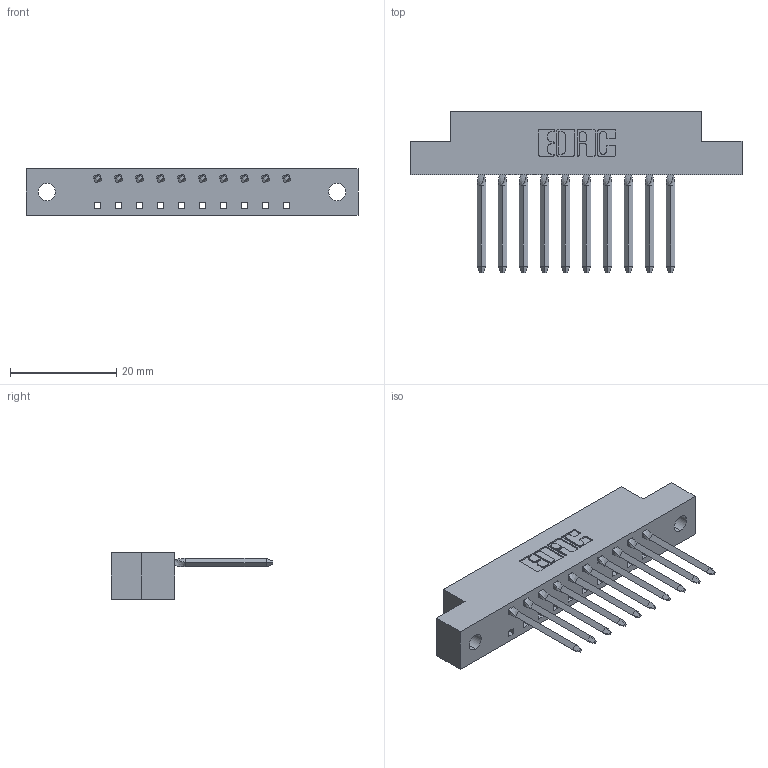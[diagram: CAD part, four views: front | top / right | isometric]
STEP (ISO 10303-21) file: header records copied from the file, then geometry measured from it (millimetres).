
FILE_DESCRIPTION (( 'STEP AP203' ), '1' );
FILE_NAME ('338-010-541-102.STEP', '2020-03-24T16:54:21', ( '' ), ( '' ), 'SwSTEP 2.0', 'SolidWorks 2016', '' );
FILE_SCHEMA (( 'CONFIG_CONTROL_DESIGN' ));
Length unit declared in the file: inch
Products named in the file (3): 338-290-001_541; 338-210-001_338-210-010-002; 338-010-541-102
Assembly tree (11 placements, depth 2):
  338-010-541-102
    338-210-001_338-210-010-002
    338-290-001_541  x10
Bounding box: 62.64 x 30.56 x 8.71 mm (x, y, z)
Volume: 4300 mm3; surface area: 6146 mm2
Topology: 11 solids, 11 shells, 1024 faces, 2821 edges, 1806 vertices
Faces by surface type: plane 700, cylinder 284, bspline 40
Entity records: 22606 total; most frequent: CARTESIAN_POINT 4614, ORIENTED_EDGE 3788, DIRECTION 3517, EDGE_CURVE 1894, VECTOR 1363, LINE 1363, VERTEX_POINT 1230, AXIS2_PLACEMENT_3D 1077
